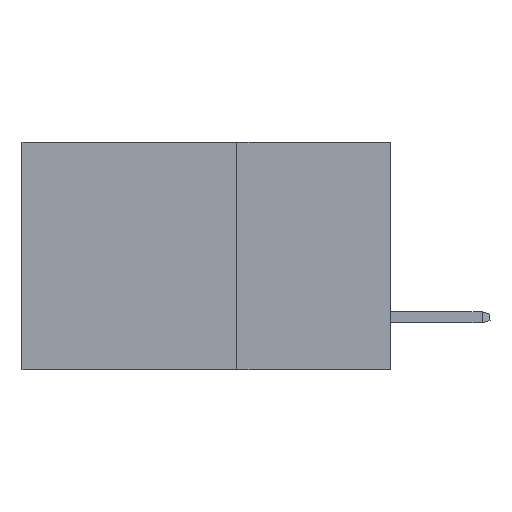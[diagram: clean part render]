
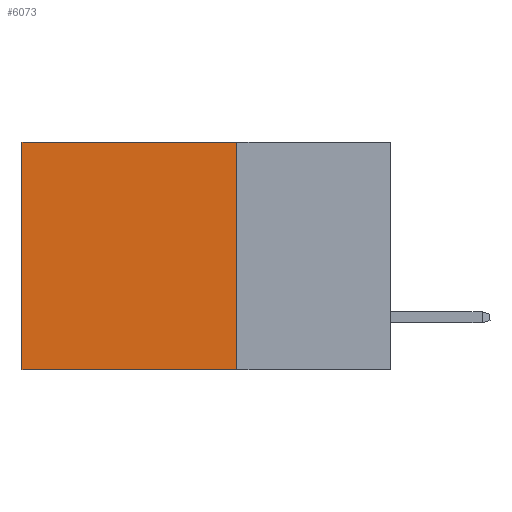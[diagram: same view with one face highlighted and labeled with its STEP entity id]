
A CAD part, left-side view. The second image highlights one B-rep face of the part: STEP entity #6073.
In plain terms, the highlighted planar face has unit normal (-1, 0, 0).
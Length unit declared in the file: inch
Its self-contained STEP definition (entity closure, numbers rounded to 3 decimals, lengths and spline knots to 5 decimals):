
#489 = VERTEX_POINT ( 'NONE', #6212 ) ;
#783 = VECTOR ( 'NONE', #2194, 39.37008 ) ;
#1020 = DIRECTION ( 'NONE',  ( 1., 0., 0. ) ) ;
#1048 = CARTESIAN_POINT ( 'NONE',  ( 0.2875, 0.6, -0.37 ) ) ;
#1620 = VERTEX_POINT ( 'NONE', #5819 ) ;
#1646 = EDGE_LOOP ( 'NONE', ( #6739, #3694, #4169, #6757 ) ) ;
#1680 = CARTESIAN_POINT ( 'NONE',  ( 0.2875, 0.25, 0. ) ) ;
#1780 = EDGE_CURVE ( 'NONE', #2030, #7998, #7028, .T. ) ;
#2030 = VERTEX_POINT ( 'NONE', #4317 ) ;
#2160 = CARTESIAN_POINT ( 'NONE',  ( 0.2875, 0.6, 0. ) ) ;
#2194 = DIRECTION ( 'NONE',  ( 0., 0., -1. ) ) ;
#2658 = VECTOR ( 'NONE', #2693, 39.37008 ) ;
#2693 = DIRECTION ( 'NONE',  ( 0., 1., 0. ) ) ;
#2798 = LINE ( 'NONE', #2160, #5448 ) ;
#3115 = PLANE ( 'NONE',  #7293 ) ;
#3694 = ORIENTED_EDGE ( 'NONE', *, *, #1780, .F. ) ;
#3746 = FACE_OUTER_BOUND ( 'NONE', #1646, .T. ) ;
#4169 = ORIENTED_EDGE ( 'NONE', *, *, #6411, .F. ) ;
#4317 = CARTESIAN_POINT ( 'NONE',  ( 0.2875, 0.25, -0.37 ) ) ;
#4322 = EDGE_CURVE ( 'NONE', #1620, #489, #6033, .T. ) ;
#4443 = DIRECTION ( 'NONE',  ( 0., 1., 0. ) ) ;
#4677 = CARTESIAN_POINT ( 'NONE',  ( 0.2875, 0.25, -0.37 ) ) ;
#5130 = DIRECTION ( 'NONE',  ( 0., 0., -1. ) ) ;
#5448 = VECTOR ( 'NONE', #5577, 39.37008 ) ;
#5577 = DIRECTION ( 'NONE',  ( 0., 0., -1. ) ) ;
#5594 = VECTOR ( 'NONE', #4443, 39.37008 ) ;
#5668 = LINE ( 'NONE', #8333, #783 ) ;
#5819 = CARTESIAN_POINT ( 'NONE',  ( 0.2875, 0.25, 0. ) ) ;
#5882 = CARTESIAN_POINT ( 'NONE',  ( 0.2875, 0.25, 0. ) ) ;
#6033 = LINE ( 'NONE', #1680, #5594 ) ;
#6073 = ADVANCED_FACE ( 'NONE', ( #3746 ), #3115, .F. ) ;
#6212 = CARTESIAN_POINT ( 'NONE',  ( 0.2875, 0.6, 0. ) ) ;
#6402 = EDGE_CURVE ( 'NONE', #489, #7998, #2798, .T. ) ;
#6411 = EDGE_CURVE ( 'NONE', #1620, #2030, #5668, .T. ) ;
#6739 = ORIENTED_EDGE ( 'NONE', *, *, #6402, .T. ) ;
#6757 = ORIENTED_EDGE ( 'NONE', *, *, #4322, .T. ) ;
#7028 = LINE ( 'NONE', #4677, #2658 ) ;
#7293 = AXIS2_PLACEMENT_3D ( 'NONE', #5882, #1020, #5130 ) ;
#7998 = VERTEX_POINT ( 'NONE', #1048 ) ;
#8333 = CARTESIAN_POINT ( 'NONE',  ( 0.2875, 0.25, 0. ) ) ;
